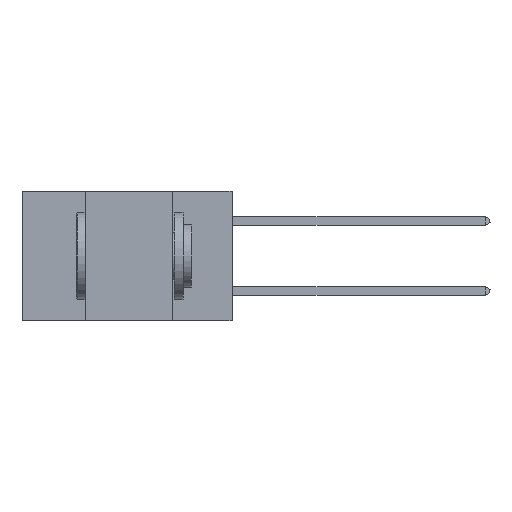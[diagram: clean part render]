
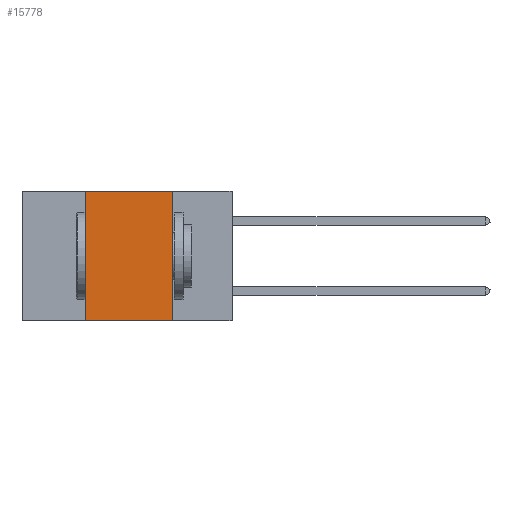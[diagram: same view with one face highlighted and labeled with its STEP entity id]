
A CAD part, left-side view. The second image highlights one B-rep face of the part: STEP entity #15778.
In plain terms, the highlighted planar face has unit normal (-1, 0, 0).
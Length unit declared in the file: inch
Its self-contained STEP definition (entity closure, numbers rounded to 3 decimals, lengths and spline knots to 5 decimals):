
#261 = CARTESIAN_POINT ( 'NONE',  ( 0., 0.6, 0. ) ) ;
#470 = CARTESIAN_POINT ( 'NONE',  ( 0., 0.42, 0. ) ) ;
#1040 = PLANE ( 'NONE',  #22929 ) ;
#1190 = FACE_OUTER_BOUND ( 'NONE', #19829, .T. ) ;
#1238 = DIRECTION ( 'NONE',  ( 0., -1., 0. ) ) ;
#1792 = VERTEX_POINT ( 'NONE', #9266 ) ;
#2988 = DIRECTION ( 'NONE',  ( 1., 0., 0. ) ) ;
#4472 = LINE ( 'NONE', #5477, #22343 ) ;
#4592 = CARTESIAN_POINT ( 'NONE',  ( 0., 0.17, -0.37 ) ) ;
#5477 = CARTESIAN_POINT ( 'NONE',  ( 0., 0.42, 0. ) ) ;
#6217 = ORIENTED_EDGE ( 'NONE', *, *, #18390, .T. ) ;
#6729 = CARTESIAN_POINT ( 'NONE',  ( 0., 0.42, -0.37 ) ) ;
#8482 = VERTEX_POINT ( 'NONE', #4592 ) ;
#8631 = CARTESIAN_POINT ( 'NONE',  ( 0., 0.6, 0. ) ) ;
#9078 = VERTEX_POINT ( 'NONE', #470 ) ;
#9266 = CARTESIAN_POINT ( 'NONE',  ( 0., 0.17, 0. ) ) ;
#9782 = DIRECTION ( 'NONE',  ( 0., -1., 0. ) ) ;
#9800 = EDGE_CURVE ( 'NONE', #1792, #8482, #18395, .T. ) ;
#10076 = ORIENTED_EDGE ( 'NONE', *, *, #15509, .F. ) ;
#11846 = LINE ( 'NONE', #261, #20923 ) ;
#12059 = DIRECTION ( 'NONE',  ( 0., 0., -1. ) ) ;
#15448 = ORIENTED_EDGE ( 'NONE', *, *, #15895, .F. ) ;
#15509 = EDGE_CURVE ( 'NONE', #9078, #1792, #11846, .T. ) ;
#15778 = ADVANCED_FACE ( 'NONE', ( #1190 ), #1040, .F. ) ;
#15895 = EDGE_CURVE ( 'NONE', #23572, #9078, #4472, .T. ) ;
#15974 = DIRECTION ( 'NONE',  ( 0., 0., -1. ) ) ;
#16160 = CARTESIAN_POINT ( 'NONE',  ( 0., 0.6, -0.37 ) ) ;
#16612 = DIRECTION ( 'NONE',  ( 0., 0., 1. ) ) ;
#17202 = VECTOR ( 'NONE', #12059, 39.37008 ) ;
#18281 = LINE ( 'NONE', #16160, #23088 ) ;
#18390 = EDGE_CURVE ( 'NONE', #23572, #8482, #18281, .T. ) ;
#18395 = LINE ( 'NONE', #22832, #17202 ) ;
#19183 = ORIENTED_EDGE ( 'NONE', *, *, #9800, .F. ) ;
#19829 = EDGE_LOOP ( 'NONE', ( #19183, #10076, #15448, #6217 ) ) ;
#20923 = VECTOR ( 'NONE', #9782, 39.37008 ) ;
#22343 = VECTOR ( 'NONE', #16612, 39.37008 ) ;
#22832 = CARTESIAN_POINT ( 'NONE',  ( 0., 0.17, 0. ) ) ;
#22929 = AXIS2_PLACEMENT_3D ( 'NONE', #8631, #2988, #15974 ) ;
#23088 = VECTOR ( 'NONE', #1238, 39.37008 ) ;
#23572 = VERTEX_POINT ( 'NONE', #6729 ) ;
